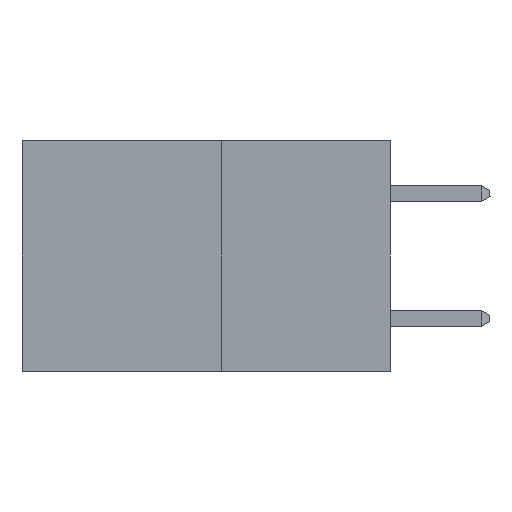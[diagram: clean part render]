
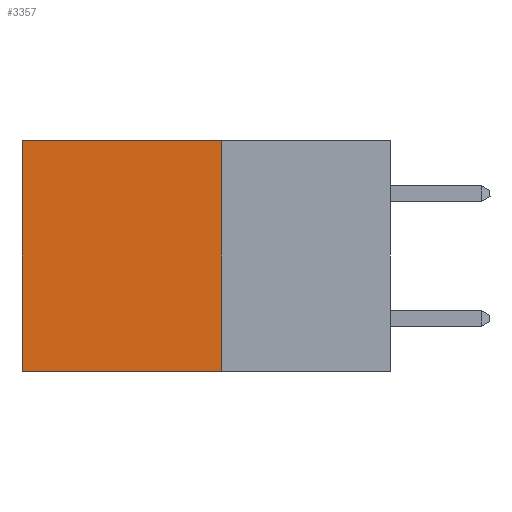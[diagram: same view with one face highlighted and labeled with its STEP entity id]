
A CAD part, left-side view. The second image highlights one B-rep face of the part: STEP entity #3357.
In plain terms, the highlighted planar face has unit normal (-1, 0, 0).
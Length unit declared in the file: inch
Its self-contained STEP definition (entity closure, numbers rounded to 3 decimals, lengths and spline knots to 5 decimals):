
#297 = DIRECTION ( 'NONE',  ( 0., 1., 0. ) ) ;
#528 = CARTESIAN_POINT ( 'NONE',  ( 0.277, 0.59, 0. ) ) ;
#593 = EDGE_CURVE ( 'NONE', #3903, #2503, #5956, .T. ) ;
#923 = DIRECTION ( 'NONE',  ( 0., 0., -1. ) ) ;
#1032 = CARTESIAN_POINT ( 'NONE',  ( 0.277, 0.27, -0.37 ) ) ;
#1114 = EDGE_LOOP ( 'NONE', ( #4849, #4985, #4603, #4481 ) ) ;
#1155 = CARTESIAN_POINT ( 'NONE',  ( 0.277, 0.27, -0.37 ) ) ;
#1613 = DIRECTION ( 'NONE',  ( 0., 1., 0. ) ) ;
#1647 = EDGE_CURVE ( 'NONE', #2076, #7746, #7388, .T. ) ;
#1726 = VECTOR ( 'NONE', #297, 39.37008 ) ;
#1995 = EDGE_CURVE ( 'NONE', #3903, #2076, #3900, .T. ) ;
#2076 = VERTEX_POINT ( 'NONE', #528 ) ;
#2078 = VECTOR ( 'NONE', #1613, 39.37008 ) ;
#2169 = CARTESIAN_POINT ( 'NONE',  ( 0.277, 0.27, 0. ) ) ;
#2339 = PLANE ( 'NONE',  #8555 ) ;
#2503 = VERTEX_POINT ( 'NONE', #8132 ) ;
#2840 = CARTESIAN_POINT ( 'NONE',  ( 0.277, 0.59, -0.37 ) ) ;
#3357 = ADVANCED_FACE ( 'NONE', ( #7611 ), #2339, .F. ) ;
#3531 = CARTESIAN_POINT ( 'NONE',  ( 0.277, 0.59, -0.37 ) ) ;
#3900 = LINE ( 'NONE', #5833, #1726 ) ;
#3903 = VERTEX_POINT ( 'NONE', #2169 ) ;
#4481 = ORIENTED_EDGE ( 'NONE', *, *, #1995, .T. ) ;
#4484 = LINE ( 'NONE', #5412, #2078 ) ;
#4603 = ORIENTED_EDGE ( 'NONE', *, *, #593, .F. ) ;
#4849 = ORIENTED_EDGE ( 'NONE', *, *, #1647, .T. ) ;
#4985 = ORIENTED_EDGE ( 'NONE', *, *, #8476, .F. ) ;
#5412 = CARTESIAN_POINT ( 'NONE',  ( 0.277, 0.27, -0.37 ) ) ;
#5732 = VECTOR ( 'NONE', #6535, 39.37008 ) ;
#5833 = CARTESIAN_POINT ( 'NONE',  ( 0.277, 0.27, 0. ) ) ;
#5956 = LINE ( 'NONE', #1155, #7410 ) ;
#6061 = DIRECTION ( 'NONE',  ( 0., 0., -1. ) ) ;
#6077 = DIRECTION ( 'NONE',  ( 1., 0., 0. ) ) ;
#6535 = DIRECTION ( 'NONE',  ( 0., 0., -1. ) ) ;
#7388 = LINE ( 'NONE', #2840, #5732 ) ;
#7410 = VECTOR ( 'NONE', #923, 39.37008 ) ;
#7611 = FACE_OUTER_BOUND ( 'NONE', #1114, .T. ) ;
#7746 = VERTEX_POINT ( 'NONE', #3531 ) ;
#8132 = CARTESIAN_POINT ( 'NONE',  ( 0.277, 0.27, -0.37 ) ) ;
#8476 = EDGE_CURVE ( 'NONE', #2503, #7746, #4484, .T. ) ;
#8555 = AXIS2_PLACEMENT_3D ( 'NONE', #1032, #6077, #6061 ) ;
